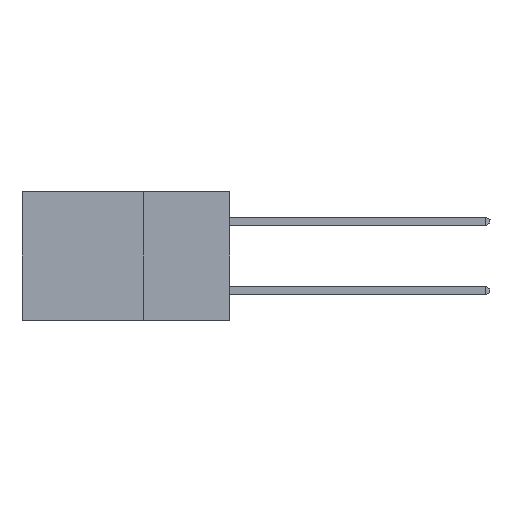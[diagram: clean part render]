
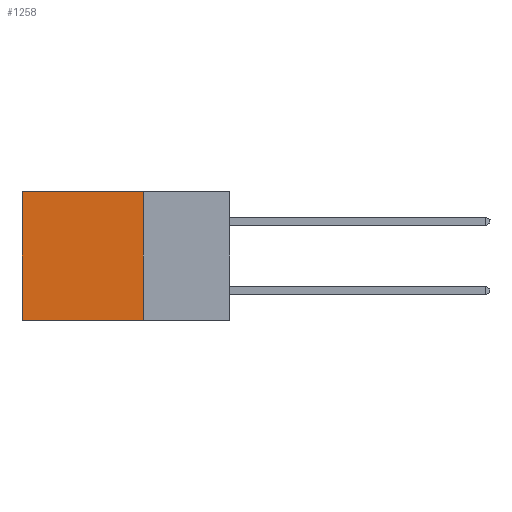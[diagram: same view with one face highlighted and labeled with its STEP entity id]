
A CAD part, left-side view. The second image highlights one B-rep face of the part: STEP entity #1258.
In plain terms, the highlighted planar face has unit normal (-1, 0, 0).
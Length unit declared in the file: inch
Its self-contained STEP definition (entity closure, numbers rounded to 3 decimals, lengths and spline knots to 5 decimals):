
#96 = ORIENTED_EDGE ( 'NONE', *, *, #22366, .T. ) ;
#1089 = LINE ( 'NONE', #10621, #14199 ) ;
#1258 = ADVANCED_FACE ( 'NONE', ( #7044 ), #25878, .F. ) ;
#2657 = CARTESIAN_POINT ( 'NONE',  ( 0.298, 0.25, 0. ) ) ;
#3898 = DIRECTION ( 'NONE',  ( 0., 0., -1. ) ) ;
#5569 = VECTOR ( 'NONE', #7102, 39.37008 ) ;
#7044 = FACE_OUTER_BOUND ( 'NONE', #10791, .T. ) ;
#7102 = DIRECTION ( 'NONE',  ( 0., 1., 0. ) ) ;
#7972 = DIRECTION ( 'NONE',  ( 1., 0., 0. ) ) ;
#9116 = VERTEX_POINT ( 'NONE', #26779 ) ;
#10204 = ORIENTED_EDGE ( 'NONE', *, *, #16998, .T. ) ;
#10519 = AXIS2_PLACEMENT_3D ( 'NONE', #21276, #7972, #23819 ) ;
#10621 = CARTESIAN_POINT ( 'NONE',  ( 0.298, 0.25, 0. ) ) ;
#10791 = EDGE_LOOP ( 'NONE', ( #10204, #16632, #11296, #96 ) ) ;
#11050 = CARTESIAN_POINT ( 'NONE',  ( 0.298, 0.6, 0. ) ) ;
#11296 = ORIENTED_EDGE ( 'NONE', *, *, #17775, .F. ) ;
#12852 = EDGE_CURVE ( 'NONE', #19298, #13717, #16318, .T. ) ;
#13405 = CARTESIAN_POINT ( 'NONE',  ( 0.298, 0.6, -0.37 ) ) ;
#13717 = VERTEX_POINT ( 'NONE', #13405 ) ;
#14199 = VECTOR ( 'NONE', #3898, 39.37008 ) ;
#14586 = VECTOR ( 'NONE', #17643, 39.37008 ) ;
#16206 = DIRECTION ( 'NONE',  ( 0., 1., 0. ) ) ;
#16318 = LINE ( 'NONE', #27346, #24363 ) ;
#16322 = VERTEX_POINT ( 'NONE', #28634 ) ;
#16324 = LINE ( 'NONE', #2657, #5569 ) ;
#16632 = ORIENTED_EDGE ( 'NONE', *, *, #12852, .F. ) ;
#16998 = EDGE_CURVE ( 'NONE', #9116, #13717, #22263, .T. ) ;
#17643 = DIRECTION ( 'NONE',  ( 0., 0., -1. ) ) ;
#17775 = EDGE_CURVE ( 'NONE', #16322, #19298, #1089, .T. ) ;
#19298 = VERTEX_POINT ( 'NONE', #26481 ) ;
#21276 = CARTESIAN_POINT ( 'NONE',  ( 0.298, 0.25, 0. ) ) ;
#22263 = LINE ( 'NONE', #11050, #14586 ) ;
#22366 = EDGE_CURVE ( 'NONE', #16322, #9116, #16324, .T. ) ;
#23819 = DIRECTION ( 'NONE',  ( 0., 0., -1. ) ) ;
#24363 = VECTOR ( 'NONE', #16206, 39.37008 ) ;
#25878 = PLANE ( 'NONE',  #10519 ) ;
#26481 = CARTESIAN_POINT ( 'NONE',  ( 0.298, 0.25, -0.37 ) ) ;
#26779 = CARTESIAN_POINT ( 'NONE',  ( 0.298, 0.6, 0. ) ) ;
#27346 = CARTESIAN_POINT ( 'NONE',  ( 0.298, 0.25, -0.37 ) ) ;
#28634 = CARTESIAN_POINT ( 'NONE',  ( 0.298, 0.25, 0. ) ) ;
